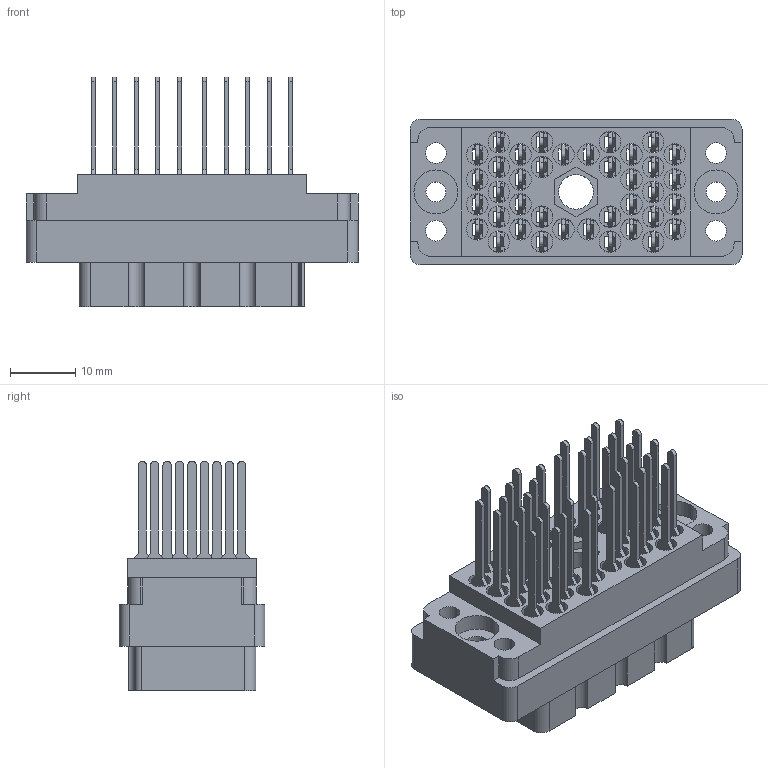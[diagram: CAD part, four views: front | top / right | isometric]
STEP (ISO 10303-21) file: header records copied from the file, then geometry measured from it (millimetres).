
FILE_DESCRIPTION (( 'STEP AP203' ), '1' );
FILE_NAME ('516-038-540-600.STEP', '2020-03-05T15:32:14', ( '' ), ( '' ), 'SwSTEP 2.0', 'SolidWorks 2016', '' );
FILE_SCHEMA (( 'CONFIG_CONTROL_DESIGN' ));
Length unit declared in the file: inch
Products named in the file (3): 516-292-001_540 Contact; 516 Part Receptacle_038; 516-038-540-600
Assembly tree (39 placements, depth 2):
  516-038-540-600
    516 Part Receptacle_038
    516-292-001_540 Contact  x38
Bounding box: 50.8 x 22.25 x 35.15 mm (x, y, z)
Volume: 12229.1 mm3; surface area: 22318.8 mm2
Topology: 39 solids, 39 shells, 3653 faces, 10600 edges, 7040 vertices
Faces by surface type: plane 2233, cylinder 1190, bspline 228, cone 2
Entity records: 34769 total; most frequent: CARTESIAN_POINT 6154, ORIENTED_EDGE 5808, DIRECTION 5669, EDGE_CURVE 2904, VECTOR 2121, LINE 2121, VERTEX_POINT 1934, AXIS2_PLACEMENT_3D 1774
